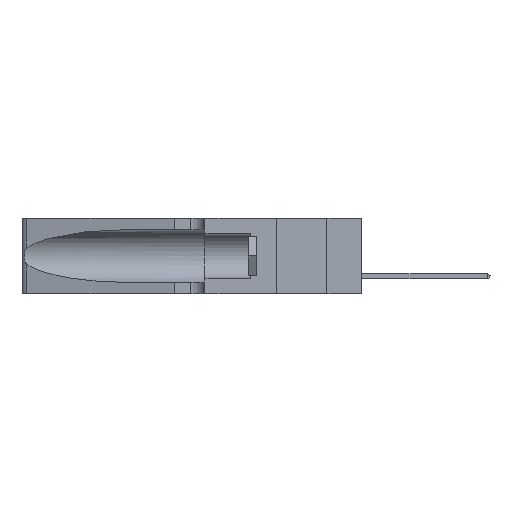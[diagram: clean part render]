
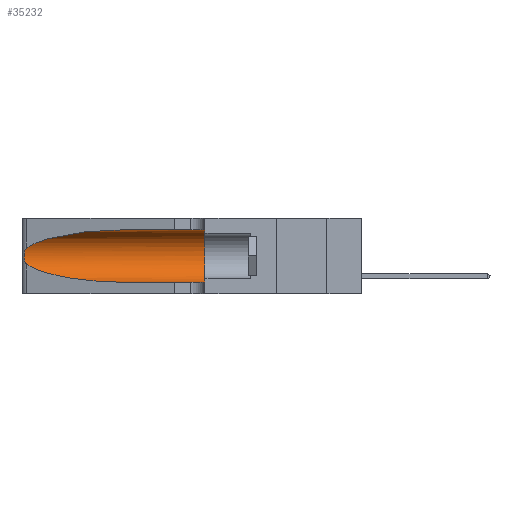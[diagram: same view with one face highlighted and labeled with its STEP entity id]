
A CAD part, left-side view. The second image highlights one B-rep face of the part: STEP entity #35232.
In plain terms, the highlighted cylindrical face has radius 3.308 mm (diameter 6.617 mm), a partial arc.
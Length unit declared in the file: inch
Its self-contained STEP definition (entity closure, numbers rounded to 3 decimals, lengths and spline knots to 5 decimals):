
#32 =( BOUNDED_CURVE ( )  B_SPLINE_CURVE ( 3, ( #35493, #1236, #23276, #16809 ),
 .UNSPECIFIED., .F., .T. ) 
 B_SPLINE_CURVE_WITH_KNOTS ( ( 4, 4 ),
 ( 3.44316, 4.71239 ),
 .UNSPECIFIED. ) 
 CURVE ( )  GEOMETRIC_REPRESENTATION_ITEM ( )  RATIONAL_B_SPLINE_CURVE ( ( 1., 0.87, 0.87, 1. ) ) 
 REPRESENTATION_ITEM ( '' )  );
#34 = VERTEX_POINT ( 'NONE', #38297 ) ;
#504 = LINE ( 'NONE', #9963, #23255 ) ;
#1236 = CARTESIAN_POINT ( 'NONE',  ( 0.2373, 1.15595, 0.08982 ) ) ;
#2064 = CARTESIAN_POINT ( 'NONE',  ( 0.25487, 1.22718, 0.22369 ) ) ;
#2339 = AXIS2_PLACEMENT_3D ( 'NONE', #2479, #6038, #2348 ) ;
#2348 = DIRECTION ( 'NONE',  ( 0., 0., -1. ) ) ;
#2479 = CARTESIAN_POINT ( 'NONE',  ( 0.1305, 1.61858, 0.185 ) ) ;
#2751 = CARTESIAN_POINT ( 'NONE',  ( 0.25555, 1.22993, 0.14849 ) ) ;
#3786 = CARTESIAN_POINT ( 'NONE',  ( 0.1305, 0.35, 0.05475 ) ) ;
#4640 = DIRECTION ( 'NONE',  ( 0., -1., 0. ) ) ;
#5240 = CARTESIAN_POINT ( 'NONE',  ( 0.1305, 0.35, 0.31525 ) ) ;
#5895 = CARTESIAN_POINT ( 'NONE',  ( 0.2373, 1.15595, 0.28018 ) ) ;
#6038 = DIRECTION ( 'NONE',  ( 0., -1., 0. ) ) ;
#6927 = LINE ( 'NONE', #14004, #39418 ) ;
#7057 = EDGE_CURVE ( 'NONE', #20964, #33782, #504, .T. ) ;
#7812 = ORIENTED_EDGE ( 'NONE', *, *, #24610, .T. ) ;
#8370 = CARTESIAN_POINT ( 'NONE',  ( 0.25555, 1.22994, 0.2215 ) ) ;
#8910 = CARTESIAN_POINT ( 'NONE',  ( 0.25639, 1.23186, 0.15144 ) ) ;
#9186 = CARTESIAN_POINT ( 'NONE',  ( 0.26017, 1.23833, 0.17102 ) ) ;
#9219 = EDGE_CURVE ( 'NONE', #33594, #34, #26978, .T. ) ;
#9963 = CARTESIAN_POINT ( 'NONE',  ( 0.1305, 1.61858, 0.05475 ) ) ;
#11592 = ORIENTED_EDGE ( 'NONE', *, *, #24862, .T. ) ;
#11602 = EDGE_CURVE ( 'NONE', #33594, #12639, #6927, .T. ) ;
#12639 = VERTEX_POINT ( 'NONE', #5240 ) ;
#13122 = CARTESIAN_POINT ( 'NONE',  ( 0.1305, 0.72297, 0.05475 ) ) ;
#13910 = ORIENTED_EDGE ( 'NONE', *, *, #9219, .T. ) ;
#14004 = CARTESIAN_POINT ( 'NONE',  ( 0.1305, 1.61858, 0.31525 ) ) ;
#14842 = CARTESIAN_POINT ( 'NONE',  ( 0.25854, 1.2359, 0.20912 ) ) ;
#15124 = CARTESIAN_POINT ( 'NONE',  ( 0.26075, 1.23896, 0.19203 ) ) ;
#15899 = B_SPLINE_CURVE_WITH_KNOTS ( 'NONE', 3,
 ( #2064, #8370, #33964, #39885, #14842, #18038, #15124, #21770, #9186, #25204, #18844, #8910, #2751, #31470 ),
 .UNSPECIFIED., .F., .F.,
 ( 4, 2, 2, 2, 2, 2, 4 ),
 ( 0., 0.00027, 0.00053, 0.00107, 0.0016, 0.00187, 0.00214 ),
 .UNSPECIFIED. ) ;
#16809 = CARTESIAN_POINT ( 'NONE',  ( 0.1305, 0.72297, 0.05475 ) ) ;
#17305 = ORIENTED_EDGE ( 'NONE', *, *, #7057, .T. ) ;
#17724 = EDGE_LOOP ( 'NONE', ( #13910, #11592, #7812, #17305, #36455, #19307 ) ) ;
#18038 = CARTESIAN_POINT ( 'NONE',  ( 0.26018, 1.23835, 0.19895 ) ) ;
#18844 = CARTESIAN_POINT ( 'NONE',  ( 0.25789, 1.23486, 0.15765 ) ) ;
#19304 = FACE_OUTER_BOUND ( 'NONE', #17724, .T. ) ;
#19307 = ORIENTED_EDGE ( 'NONE', *, *, #11602, .F. ) ;
#20964 = VERTEX_POINT ( 'NONE', #13122 ) ;
#21760 = CARTESIAN_POINT ( 'NONE',  ( 0.18966, 0.96281, 0.31525 ) ) ;
#21770 = CARTESIAN_POINT ( 'NONE',  ( 0.26075, 1.23896, 0.178 ) ) ;
#22632 = DIRECTION ( 'NONE',  ( 0., -1., 0. ) ) ;
#23255 = VECTOR ( 'NONE', #22632, 39.37008 ) ;
#23276 = CARTESIAN_POINT ( 'NONE',  ( 0.18966, 0.96281, 0.05475 ) ) ;
#24610 = EDGE_CURVE ( 'NONE', #37276, #20964, #32, .T. ) ;
#24862 = EDGE_CURVE ( 'NONE', #34, #37276, #15899, .T. ) ;
#25204 = CARTESIAN_POINT ( 'NONE',  ( 0.25856, 1.23593, 0.16098 ) ) ;
#25707 = CARTESIAN_POINT ( 'NONE',  ( 0.1305, 0.72297, 0.31525 ) ) ;
#26908 = DIRECTION ( 'NONE',  ( 0., 0., 1. ) ) ;
#26978 =( BOUNDED_CURVE ( )  B_SPLINE_CURVE ( 3, ( #30932, #21760, #5895, #27926 ),
 .UNSPECIFIED., .F., .T. ) 
 B_SPLINE_CURVE_WITH_KNOTS ( ( 4, 4 ),
 ( 1.5708, 2.84003 ),
 .UNSPECIFIED. ) 
 CURVE ( )  GEOMETRIC_REPRESENTATION_ITEM ( )  RATIONAL_B_SPLINE_CURVE ( ( 1., 0.87, 0.87, 1. ) ) 
 REPRESENTATION_ITEM ( '' )  );
#27926 = CARTESIAN_POINT ( 'NONE',  ( 0.25487, 1.22718, 0.22369 ) ) ;
#30526 = AXIS2_PLACEMENT_3D ( 'NONE', #39012, #39154, #26908 ) ;
#30932 = CARTESIAN_POINT ( 'NONE',  ( 0.1305, 0.72297, 0.31525 ) ) ;
#31470 = CARTESIAN_POINT ( 'NONE',  ( 0.25487, 1.22718, 0.14631 ) ) ;
#33102 = CARTESIAN_POINT ( 'NONE',  ( 0.25487, 1.22718, 0.14631 ) ) ;
#33515 = CIRCLE ( 'NONE', #30526, 0.13025 ) ;
#33594 = VERTEX_POINT ( 'NONE', #25707 ) ;
#33782 = VERTEX_POINT ( 'NONE', #3786 ) ;
#33964 = CARTESIAN_POINT ( 'NONE',  ( 0.25639, 1.23184, 0.21858 ) ) ;
#35232 = ADVANCED_FACE ( 'NONE', ( #19304 ), #39470, .F. ) ;
#35493 = CARTESIAN_POINT ( 'NONE',  ( 0.25487, 1.22718, 0.14631 ) ) ;
#35711 = EDGE_CURVE ( 'NONE', #12639, #33782, #33515, .T. ) ;
#36455 = ORIENTED_EDGE ( 'NONE', *, *, #35711, .F. ) ;
#37276 = VERTEX_POINT ( 'NONE', #33102 ) ;
#38297 = CARTESIAN_POINT ( 'NONE',  ( 0.25487, 1.22718, 0.22369 ) ) ;
#39012 = CARTESIAN_POINT ( 'NONE',  ( 0.1305, 0.35, 0.185 ) ) ;
#39154 = DIRECTION ( 'NONE',  ( 0., 1., 0. ) ) ;
#39418 = VECTOR ( 'NONE', #4640, 39.37008 ) ;
#39470 = CYLINDRICAL_SURFACE ( 'NONE', #2339, 0.13025 ) ;
#39885 = CARTESIAN_POINT ( 'NONE',  ( 0.25787, 1.23484, 0.2124 ) ) ;
